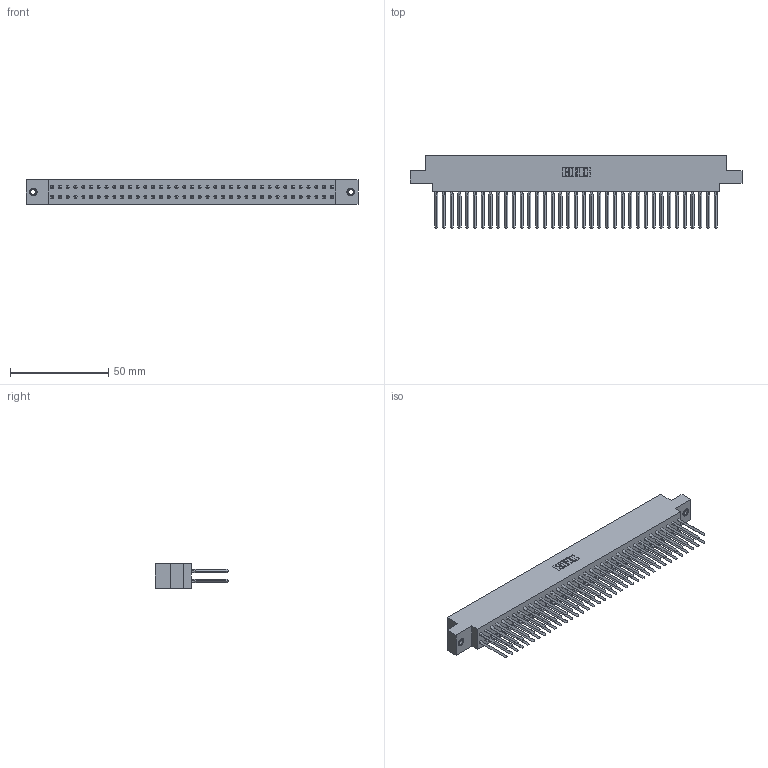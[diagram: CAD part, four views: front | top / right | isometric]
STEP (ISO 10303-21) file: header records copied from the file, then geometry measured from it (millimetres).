
FILE_DESCRIPTION (( 'STEP AP203' ), '1' );
FILE_NAME ('317-074-542-807.STEP', '2020-02-28T07:59:45', ( '' ), ( '' ), 'SwSTEP 2.0', 'SolidWorks 2016', '' );
FILE_SCHEMA (( 'CONFIG_CONTROL_DESIGN' ));
Length unit declared in the file: inch
Products named in the file (4): 317-290-003_542; 317-074-542-807; 317 Part_.156 Dia - TI; 345-250-001_345-250-005-103
Assembly tree (77 placements, depth 2):
  317-074-542-807
    317 Part_.156 Dia - TI
    317-290-003_542  x74
    345-250-001_345-250-005-103  x2
Bounding box: 169.32 x 37.34 x 12.7 mm (x, y, z)
Volume: 27553.5 mm3; surface area: 38191.5 mm2
Topology: 77 solids, 77 shells, 4380 faces, 12251 edges, 7814 vertices
Faces by surface type: plane 3494, cylinder 574, bspline 296, cone 12, torus 4
Entity records: 54384 total; most frequent: CARTESIAN_POINT 9708, ORIENTED_EDGE 9364, DIRECTION 7924, EDGE_CURVE 4682, VECTOR 4492, LINE 4492, VERTEX_POINT 3112, AXIS2_PLACEMENT_3D 1716
